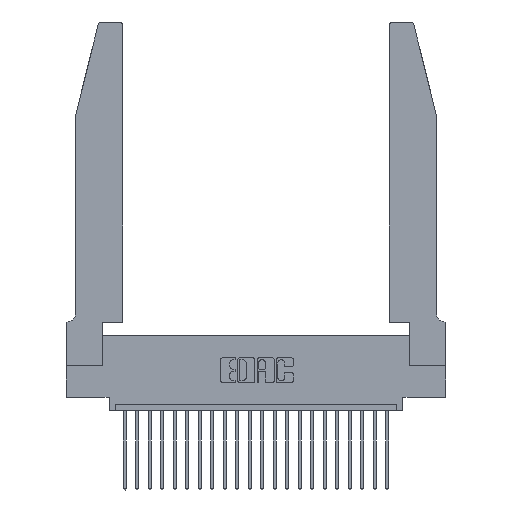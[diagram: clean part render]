
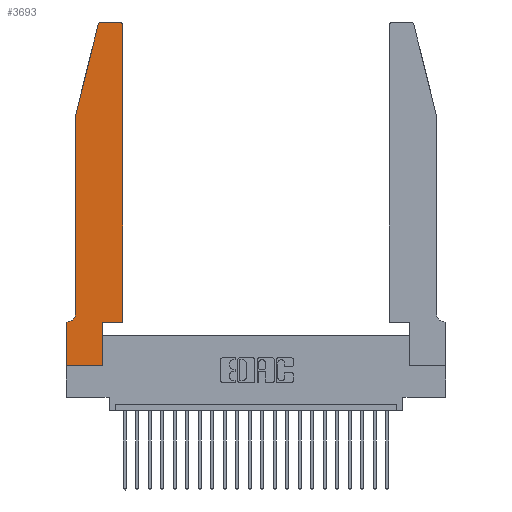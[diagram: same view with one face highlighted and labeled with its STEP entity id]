
A CAD part, top view. The second image highlights one B-rep face of the part: STEP entity #3693.
In plain terms, the highlighted planar face has unit normal (0, 0, 1).
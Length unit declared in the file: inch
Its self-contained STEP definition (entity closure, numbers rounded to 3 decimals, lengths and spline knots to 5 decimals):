
#361 = DIRECTION ( 'NONE',  ( 1., 0., 0. ) ) ;
#366 = ORIENTED_EDGE ( 'NONE', *, *, #4962, .T. ) ;
#917 = DIRECTION ( 'NONE',  ( 0., -1., 0. ) ) ;
#1174 = VERTEX_POINT ( 'NONE', #13996 ) ;
#1428 = EDGE_CURVE ( 'NONE', #8279, #7483, #2200, .T. ) ;
#1519 = VECTOR ( 'NONE', #917, 39.37008 ) ;
#1969 = CIRCLE ( 'NONE', #4644, 0.07 ) ;
#1978 = ORIENTED_EDGE ( 'NONE', *, *, #2784, .T. ) ;
#2000 = LINE ( 'NONE', #14902, #8971 ) ;
#2158 = EDGE_CURVE ( 'NONE', #19594, #4932, #7115, .T. ) ;
#2200 = LINE ( 'NONE', #20859, #17692 ) ;
#2419 = ORIENTED_EDGE ( 'NONE', *, *, #13696, .T. ) ;
#2738 = LINE ( 'NONE', #23441, #11180 ) ;
#2784 = EDGE_CURVE ( 'NONE', #16058, #19529, #2738, .T. ) ;
#2856 = DIRECTION ( 'NONE',  ( 0., 1., 0. ) ) ;
#2926 = VERTEX_POINT ( 'NONE', #21983 ) ;
#3235 = DIRECTION ( 'NONE',  ( 0., 1., 0. ) ) ;
#3285 = CARTESIAN_POINT ( 'NONE',  ( 0.4205, 2.75, 0.37 ) ) ;
#3502 = CARTESIAN_POINT ( 'NONE',  ( 0.0055, 0.42, 0.37 ) ) ;
#3643 = EDGE_CURVE ( 'NONE', #7483, #14038, #6204, .T. ) ;
#3651 = CARTESIAN_POINT ( 'NONE',  ( 0.2865, 0.35, 0.37 ) ) ;
#3662 = ORIENTED_EDGE ( 'NONE', *, *, #18184, .T. ) ;
#3693 = ADVANCED_FACE ( 'NONE', ( #13219 ), #18685, .T. ) ;
#4268 = DIRECTION ( 'NONE',  ( 1., 0., 0. ) ) ;
#4485 = CARTESIAN_POINT ( 'NONE',  ( 0.284, 2.75, 0.37 ) ) ;
#4533 = DIRECTION ( 'NONE',  ( 1., 0., 0. ) ) ;
#4644 = AXIS2_PLACEMENT_3D ( 'NONE', #3502, #11065, #9410 ) ;
#4932 = VERTEX_POINT ( 'NONE', #5891 ) ;
#4962 = EDGE_CURVE ( 'NONE', #19529, #19594, #13463, .T. ) ;
#5246 = CARTESIAN_POINT ( 'NONE',  ( 0.2865, 0.35, 0.37 ) ) ;
#5776 = ORIENTED_EDGE ( 'NONE', *, *, #1428, .T. ) ;
#5891 = CARTESIAN_POINT ( 'NONE',  ( 0.0755, 2., 0.37 ) ) ;
#6204 = LINE ( 'NONE', #5246, #13536 ) ;
#6663 = DIRECTION ( 'NONE',  ( -1., 0., 0. ) ) ;
#6898 = EDGE_CURVE ( 'NONE', #10810, #8279, #18695, .T. ) ;
#6947 = CARTESIAN_POINT ( 'NONE',  ( 0.0755, 0.42, 0.37 ) ) ;
#7115 = LINE ( 'NONE', #19247, #23494 ) ;
#7483 = VERTEX_POINT ( 'NONE', #7589 ) ;
#7589 = CARTESIAN_POINT ( 'NONE',  ( 0.2865, 0., 0.37 ) ) ;
#8279 = VERTEX_POINT ( 'NONE', #14515 ) ;
#8374 = CARTESIAN_POINT ( 'NONE',  ( 0.0755, 2., 0.37 ) ) ;
#8878 = EDGE_CURVE ( 'NONE', #20641, #16058, #13052, .T. ) ;
#8971 = VECTOR ( 'NONE', #14213, 39.37008 ) ;
#9410 = DIRECTION ( 'NONE',  ( -1., 0., 0. ) ) ;
#9805 = VECTOR ( 'NONE', #10999, 39.37008 ) ;
#9914 = DIRECTION ( 'NONE',  ( -0.239, -0.971, 0. ) ) ;
#10100 = ORIENTED_EDGE ( 'NONE', *, *, #3643, .T. ) ;
#10288 = AXIS2_PLACEMENT_3D ( 'NONE', #12994, #13081, #14948 ) ;
#10810 = VERTEX_POINT ( 'NONE', #13421 ) ;
#10999 = DIRECTION ( 'NONE',  ( -1., 0., 0. ) ) ;
#11065 = DIRECTION ( 'NONE',  ( 0., 0., -1. ) ) ;
#11180 = VECTOR ( 'NONE', #6663, 39.37008 ) ;
#11604 = DIRECTION ( 'NONE',  ( 0., 0., 1. ) ) ;
#11739 = AXIS2_PLACEMENT_3D ( 'NONE', #13330, #11604, #4268 ) ;
#12023 = LINE ( 'NONE', #8374, #1519 ) ;
#12212 = CARTESIAN_POINT ( 'NONE',  ( 0.0755, 0.35, 0.37 ) ) ;
#12508 = ORIENTED_EDGE ( 'NONE', *, *, #14040, .T. ) ;
#12585 = VECTOR ( 'NONE', #22487, 39.37008 ) ;
#12994 = CARTESIAN_POINT ( 'NONE',  ( 0., 0.35, 0.37 ) ) ;
#13052 = CIRCLE ( 'NONE', #20875, 0.03 ) ;
#13081 = DIRECTION ( 'NONE',  ( 0., 0., 1. ) ) ;
#13219 = FACE_OUTER_BOUND ( 'NONE', #16807, .T. ) ;
#13330 = CARTESIAN_POINT ( 'NONE',  ( 0.284, 2.72, 0.37 ) ) ;
#13421 = CARTESIAN_POINT ( 'NONE',  ( 0., 0.35, 0.37 ) ) ;
#13463 = CIRCLE ( 'NONE', #11739, 0.03 ) ;
#13536 = VECTOR ( 'NONE', #3235, 39.37008 ) ;
#13696 = EDGE_CURVE ( 'NONE', #23846, #1174, #1969, .T. ) ;
#13951 = LINE ( 'NONE', #12212, #9805 ) ;
#13996 = CARTESIAN_POINT ( 'NONE',  ( 0.0055, 0.35, 0.37 ) ) ;
#14038 = VERTEX_POINT ( 'NONE', #3651 ) ;
#14040 = EDGE_CURVE ( 'NONE', #14038, #2926, #2000, .T. ) ;
#14108 = CARTESIAN_POINT ( 'NONE',  ( 0.25487, 2.72718, 0.37 ) ) ;
#14194 = LINE ( 'NONE', #15831, #15642 ) ;
#14213 = DIRECTION ( 'NONE',  ( 1., 0., 0. ) ) ;
#14515 = CARTESIAN_POINT ( 'NONE',  ( 0., 0., 0.37 ) ) ;
#14681 = EDGE_CURVE ( 'NONE', #1174, #10810, #13951, .T. ) ;
#14902 = CARTESIAN_POINT ( 'NONE',  ( 0.4505, 0.35, 0.37 ) ) ;
#14916 = ORIENTED_EDGE ( 'NONE', *, *, #2158, .T. ) ;
#14948 = DIRECTION ( 'NONE',  ( 1., 0., 0. ) ) ;
#15547 = ORIENTED_EDGE ( 'NONE', *, *, #6898, .T. ) ;
#15642 = VECTOR ( 'NONE', #2856, 39.37008 ) ;
#15713 = DIRECTION ( 'NONE',  ( 0., 0., 1. ) ) ;
#15831 = CARTESIAN_POINT ( 'NONE',  ( 0.4505, 0.35, 0.37 ) ) ;
#15926 = ORIENTED_EDGE ( 'NONE', *, *, #23074, .T. ) ;
#16058 = VERTEX_POINT ( 'NONE', #3285 ) ;
#16807 = EDGE_LOOP ( 'NONE', ( #1978, #366, #14916, #3662, #2419, #22256, #15547, #5776, #10100, #12508, #15926, #19910 ) ) ;
#17692 = VECTOR ( 'NONE', #361, 39.37008 ) ;
#18184 = EDGE_CURVE ( 'NONE', #4932, #23846, #12023, .T. ) ;
#18685 = PLANE ( 'NONE',  #10288 ) ;
#18695 = LINE ( 'NONE', #21751, #12585 ) ;
#19247 = CARTESIAN_POINT ( 'NONE',  ( 0.0755, 2., 0.37 ) ) ;
#19529 = VERTEX_POINT ( 'NONE', #4485 ) ;
#19594 = VERTEX_POINT ( 'NONE', #14108 ) ;
#19910 = ORIENTED_EDGE ( 'NONE', *, *, #8878, .T. ) ;
#20641 = VERTEX_POINT ( 'NONE', #21244 ) ;
#20859 = CARTESIAN_POINT ( 'NONE',  ( 0., 0., 0.37 ) ) ;
#20875 = AXIS2_PLACEMENT_3D ( 'NONE', #21223, #15713, #4533 ) ;
#21223 = CARTESIAN_POINT ( 'NONE',  ( 0.4205, 2.72, 0.37 ) ) ;
#21244 = CARTESIAN_POINT ( 'NONE',  ( 0.4505, 2.72, 0.37 ) ) ;
#21751 = CARTESIAN_POINT ( 'NONE',  ( 0., 0., 0.37 ) ) ;
#21983 = CARTESIAN_POINT ( 'NONE',  ( 0.4505, 0.35, 0.37 ) ) ;
#22256 = ORIENTED_EDGE ( 'NONE', *, *, #14681, .T. ) ;
#22487 = DIRECTION ( 'NONE',  ( 0., -1., 0. ) ) ;
#23074 = EDGE_CURVE ( 'NONE', #2926, #20641, #14194, .T. ) ;
#23441 = CARTESIAN_POINT ( 'NONE',  ( 0.2605, 2.75, 0.37 ) ) ;
#23494 = VECTOR ( 'NONE', #9914, 39.37008 ) ;
#23846 = VERTEX_POINT ( 'NONE', #6947 ) ;
